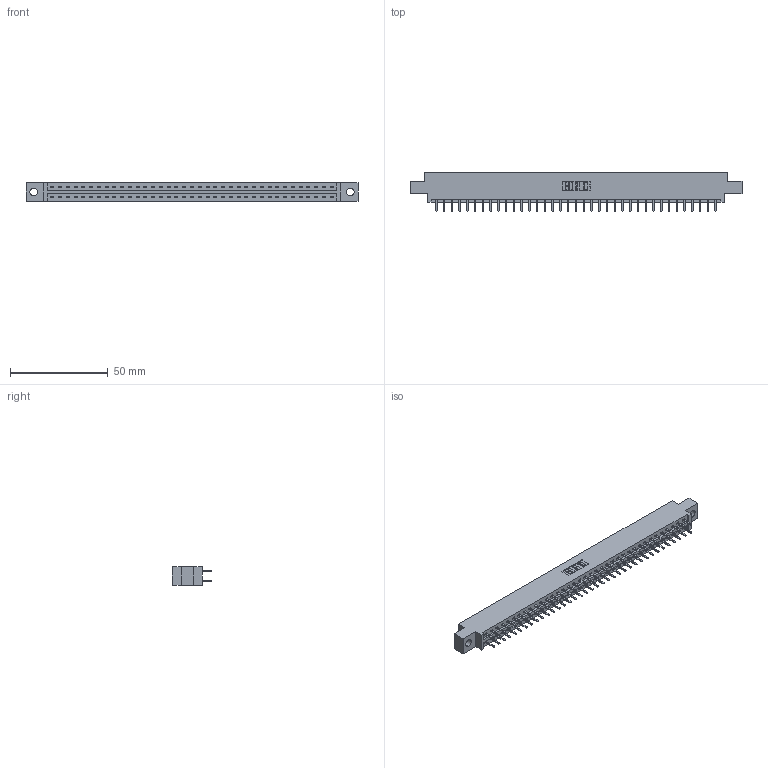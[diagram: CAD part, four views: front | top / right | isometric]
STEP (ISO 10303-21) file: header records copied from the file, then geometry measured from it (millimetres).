
FILE_DESCRIPTION (( 'STEP AP203' ), '1' );
FILE_NAME ('337-074-520-804.STEP', '2018-08-11T16:32:13', ( '' ), ( '' ), 'SwSTEP 2.0', 'SolidWorks 2016', '' );
FILE_SCHEMA (( 'CONFIG_CONTROL_DESIGN' ));
Length unit declared in the file: inch
Products named in the file (3): 345-292-001_345-293-120; 337-074-520-804; 337 Part_0.170 Offset - 0.156 Dia-TH
Assembly tree (75 placements, depth 2):
  337-074-520-804
    337 Part_0.170 Offset - 0.156 Dia-TH
    345-292-001_345-293-120  x74
Bounding box: 169.62 x 20.02 x 9.4 mm (x, y, z)
Volume: 17571.6 mm3; surface area: 19628.6 mm2
Topology: 75 solids, 75 shells, 4410 faces, 12829 edges, 8354 vertices
Faces by surface type: plane 3034, cylinder 1376
Entity records: 29583 total; most frequent: CARTESIAN_POINT 5002, ORIENTED_EDGE 4926, DIRECTION 4251, EDGE_CURVE 2463, VECTOR 2331, LINE 2331, VERTEX_POINT 1638, AXIS2_PLACEMENT_3D 960
